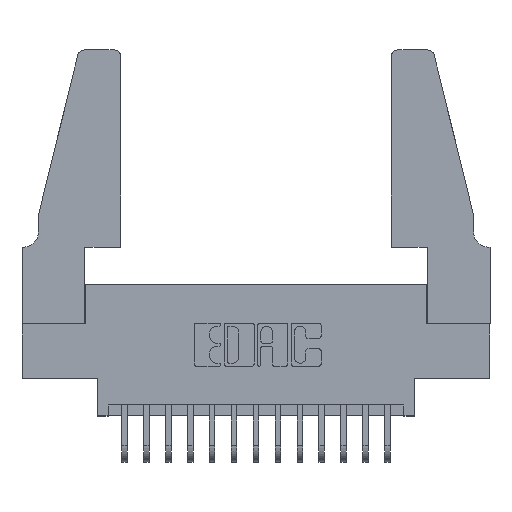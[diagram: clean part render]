
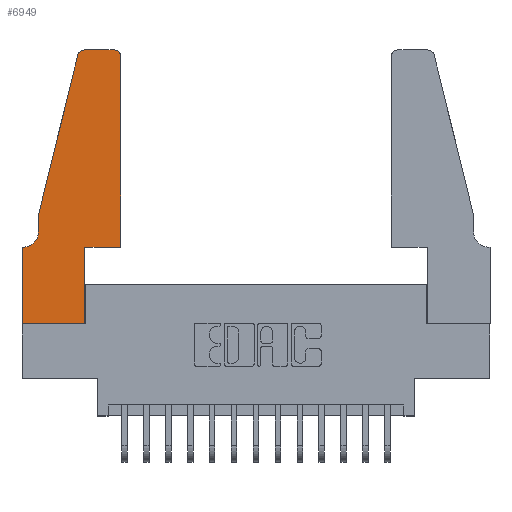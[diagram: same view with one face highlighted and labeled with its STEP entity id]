
A CAD part, top view. The second image highlights one B-rep face of the part: STEP entity #6949.
In plain terms, the highlighted planar face has unit normal (0, 0, 1).
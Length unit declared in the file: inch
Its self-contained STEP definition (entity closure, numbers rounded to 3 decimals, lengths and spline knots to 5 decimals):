
#38 = CARTESIAN_POINT ( 'NONE',  ( 0.4505, 1.22, 0.37 ) ) ;
#413 = CARTESIAN_POINT ( 'NONE',  ( 0.4505, 0.35, 0.37 ) ) ;
#519 = CARTESIAN_POINT ( 'NONE',  ( 0.0755, 0.35, 0.37 ) ) ;
#682 = AXIS2_PLACEMENT_3D ( 'NONE', #9082, #1863, #12965 ) ;
#724 = VECTOR ( 'NONE', #17721, 39.37008 ) ;
#1069 = CARTESIAN_POINT ( 'NONE',  ( 0.0055, 0.35, 0.37 ) ) ;
#1183 = LINE ( 'NONE', #9261, #724 ) ;
#1370 = EDGE_CURVE ( 'NONE', #2657, #8644, #1858, .T. ) ;
#1823 = DIRECTION ( 'NONE',  ( -1., 0., 0. ) ) ;
#1858 = LINE ( 'NONE', #519, #3155 ) ;
#1863 = DIRECTION ( 'NONE',  ( 0., 0., 1. ) ) ;
#2041 = CIRCLE ( 'NONE', #682, 0.03 ) ;
#2069 = DIRECTION ( 'NONE',  ( 1., 0., 0. ) ) ;
#2341 = FACE_OUTER_BOUND ( 'NONE', #14902, .T. ) ;
#2509 = EDGE_CURVE ( 'NONE', #11541, #5278, #12054, .T. ) ;
#2544 = VERTEX_POINT ( 'NONE', #12085 ) ;
#2650 = CARTESIAN_POINT ( 'NONE',  ( 0.4205, 1.22, 0.37 ) ) ;
#2657 = VERTEX_POINT ( 'NONE', #1069 ) ;
#2964 = CARTESIAN_POINT ( 'NONE',  ( 0.0755, 0.5, 0.37 ) ) ;
#3155 = VECTOR ( 'NONE', #1823, 39.37008 ) ;
#3165 = EDGE_CURVE ( 'NONE', #11506, #13853, #7621, .T. ) ;
#3746 = VECTOR ( 'NONE', #10189, 39.37008 ) ;
#3955 = VERTEX_POINT ( 'NONE', #38 ) ;
#4070 = EDGE_CURVE ( 'NONE', #2544, #2657, #8498, .T. ) ;
#4490 = CARTESIAN_POINT ( 'NONE',  ( 0.25487, 1.22718, 0.37 ) ) ;
#4549 = ORIENTED_EDGE ( 'NONE', *, *, #12272, .T. ) ;
#4633 = CIRCLE ( 'NONE', #11989, 0.03 ) ;
#4775 = CARTESIAN_POINT ( 'NONE',  ( 0., 0.35, 0.37 ) ) ;
#4811 = VECTOR ( 'NONE', #13203, 39.37008 ) ;
#5217 = LINE ( 'NONE', #9873, #8463 ) ;
#5278 = VERTEX_POINT ( 'NONE', #8256 ) ;
#5306 = DIRECTION ( 'NONE',  ( 0., 0., 1. ) ) ;
#5316 = EDGE_CURVE ( 'NONE', #14849, #10384, #5217, .T. ) ;
#5382 = AXIS2_PLACEMENT_3D ( 'NONE', #4775, #9052, #10414 ) ;
#5404 = VERTEX_POINT ( 'NONE', #413 ) ;
#5936 = ORIENTED_EDGE ( 'NONE', *, *, #13844, .T. ) ;
#6949 = ADVANCED_FACE ( 'NONE', ( #2341 ), #15800, .T. ) ;
#7123 = CARTESIAN_POINT ( 'NONE',  ( 0.4505, 0.35, 0.37 ) ) ;
#7536 = LINE ( 'NONE', #7123, #8873 ) ;
#7621 = LINE ( 'NONE', #2964, #16853 ) ;
#7772 = EDGE_CURVE ( 'NONE', #5278, #8275, #10700, .T. ) ;
#7785 = CARTESIAN_POINT ( 'NONE',  ( 0., 0., 0.37 ) ) ;
#8056 = ORIENTED_EDGE ( 'NONE', *, *, #13078, .T. ) ;
#8256 = CARTESIAN_POINT ( 'NONE',  ( 0.2865, 0., 0.37 ) ) ;
#8275 = VERTEX_POINT ( 'NONE', #14271 ) ;
#8396 = ORIENTED_EDGE ( 'NONE', *, *, #7772, .T. ) ;
#8463 = VECTOR ( 'NONE', #9808, 39.37008 ) ;
#8498 = CIRCLE ( 'NONE', #11206, 0.07 ) ;
#8644 = VERTEX_POINT ( 'NONE', #16969 ) ;
#8873 = VECTOR ( 'NONE', #12569, 39.37008 ) ;
#8950 = CARTESIAN_POINT ( 'NONE',  ( 0.4505, 0.35, 0.37 ) ) ;
#9052 = DIRECTION ( 'NONE',  ( 0., 0., 1. ) ) ;
#9082 = CARTESIAN_POINT ( 'NONE',  ( 0.284, 1.22, 0.37 ) ) ;
#9261 = CARTESIAN_POINT ( 'NONE',  ( 0.0755, 0.5, 0.37 ) ) ;
#9808 = DIRECTION ( 'NONE',  ( -1., 0., 0. ) ) ;
#9873 = CARTESIAN_POINT ( 'NONE',  ( 0.2605, 1.25, 0.37 ) ) ;
#9926 = ORIENTED_EDGE ( 'NONE', *, *, #2509, .T. ) ;
#10065 = LINE ( 'NONE', #8950, #3746 ) ;
#10189 = DIRECTION ( 'NONE',  ( 0., 1., 0. ) ) ;
#10191 = EDGE_CURVE ( 'NONE', #8275, #5404, #7536, .T. ) ;
#10244 = CARTESIAN_POINT ( 'NONE',  ( 0.0755, 0.5, 0.37 ) ) ;
#10384 = VERTEX_POINT ( 'NONE', #17118 ) ;
#10391 = DIRECTION ( 'NONE',  ( 0., 1., 0. ) ) ;
#10414 = DIRECTION ( 'NONE',  ( 1., 0., 0. ) ) ;
#10435 = DIRECTION ( 'NONE',  ( -1., 0., 0. ) ) ;
#10700 = LINE ( 'NONE', #16556, #14118 ) ;
#10935 = ORIENTED_EDGE ( 'NONE', *, *, #5316, .T. ) ;
#10942 = DIRECTION ( 'NONE',  ( 1., 0., 0. ) ) ;
#11060 = ORIENTED_EDGE ( 'NONE', *, *, #1370, .T. ) ;
#11206 = AXIS2_PLACEMENT_3D ( 'NONE', #16012, #17471, #10435 ) ;
#11419 = DIRECTION ( 'NONE',  ( -0.239, -0.971, 0. ) ) ;
#11506 = VERTEX_POINT ( 'NONE', #4490 ) ;
#11541 = VERTEX_POINT ( 'NONE', #15626 ) ;
#11766 = ORIENTED_EDGE ( 'NONE', *, *, #13789, .T. ) ;
#11989 = AXIS2_PLACEMENT_3D ( 'NONE', #2650, #5306, #10942 ) ;
#12054 = LINE ( 'NONE', #7785, #13984 ) ;
#12085 = CARTESIAN_POINT ( 'NONE',  ( 0.0755, 0.42, 0.37 ) ) ;
#12272 = EDGE_CURVE ( 'NONE', #3955, #14849, #4633, .T. ) ;
#12350 = ORIENTED_EDGE ( 'NONE', *, *, #3165, .T. ) ;
#12569 = DIRECTION ( 'NONE',  ( 1., 0., 0. ) ) ;
#12965 = DIRECTION ( 'NONE',  ( 1., 0., 0. ) ) ;
#13078 = EDGE_CURVE ( 'NONE', #10384, #11506, #2041, .T. ) ;
#13110 = EDGE_CURVE ( 'NONE', #13853, #2544, #1183, .T. ) ;
#13203 = DIRECTION ( 'NONE',  ( 0., -1., 0. ) ) ;
#13789 = EDGE_CURVE ( 'NONE', #5404, #3955, #10065, .T. ) ;
#13844 = EDGE_CURVE ( 'NONE', #8644, #11541, #17938, .T. ) ;
#13853 = VERTEX_POINT ( 'NONE', #10244 ) ;
#13984 = VECTOR ( 'NONE', #2069, 39.37008 ) ;
#14118 = VECTOR ( 'NONE', #10391, 39.37008 ) ;
#14237 = ORIENTED_EDGE ( 'NONE', *, *, #13110, .T. ) ;
#14271 = CARTESIAN_POINT ( 'NONE',  ( 0.2865, 0.35, 0.37 ) ) ;
#14849 = VERTEX_POINT ( 'NONE', #16997 ) ;
#14902 = EDGE_LOOP ( 'NONE', ( #10935, #8056, #12350, #14237, #14999, #11060, #5936, #9926, #8396, #16193, #11766, #4549 ) ) ;
#14999 = ORIENTED_EDGE ( 'NONE', *, *, #4070, .T. ) ;
#15626 = CARTESIAN_POINT ( 'NONE',  ( 0., 0., 0.37 ) ) ;
#15800 = PLANE ( 'NONE',  #5382 ) ;
#15950 = CARTESIAN_POINT ( 'NONE',  ( 0., 0., 0.37 ) ) ;
#16012 = CARTESIAN_POINT ( 'NONE',  ( 0.0055, 0.42, 0.37 ) ) ;
#16193 = ORIENTED_EDGE ( 'NONE', *, *, #10191, .T. ) ;
#16556 = CARTESIAN_POINT ( 'NONE',  ( 0.2865, 0.35, 0.37 ) ) ;
#16853 = VECTOR ( 'NONE', #11419, 39.37008 ) ;
#16969 = CARTESIAN_POINT ( 'NONE',  ( 0., 0.35, 0.37 ) ) ;
#16997 = CARTESIAN_POINT ( 'NONE',  ( 0.4205, 1.25, 0.37 ) ) ;
#17118 = CARTESIAN_POINT ( 'NONE',  ( 0.284, 1.25, 0.37 ) ) ;
#17471 = DIRECTION ( 'NONE',  ( 0., 0., -1. ) ) ;
#17721 = DIRECTION ( 'NONE',  ( 0., -1., 0. ) ) ;
#17938 = LINE ( 'NONE', #15950, #4811 ) ;
